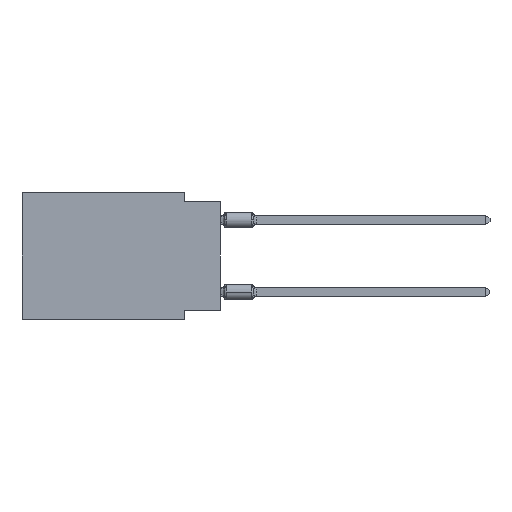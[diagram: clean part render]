
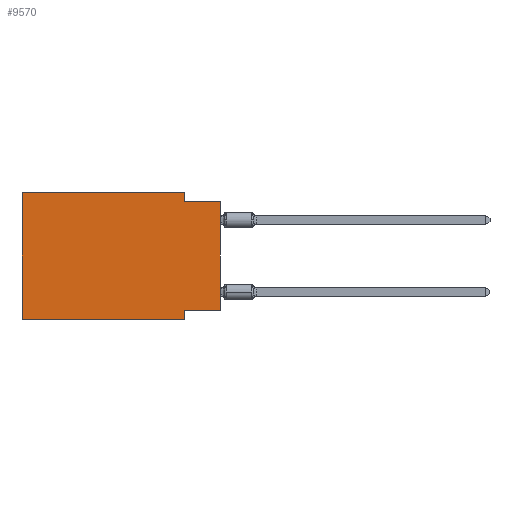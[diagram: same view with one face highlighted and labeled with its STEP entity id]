
A CAD part, left-side view. The second image highlights one B-rep face of the part: STEP entity #9570.
In plain terms, the highlighted planar face has unit normal (-1, 0, 0).
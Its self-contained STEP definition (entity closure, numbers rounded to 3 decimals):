
#768 = CARTESIAN_POINT ( 'NONE',  ( 0., 13.97, 0. ) ) ;
#900 = CARTESIAN_POINT ( 'NONE',  ( 0., 2.54, 0. ) ) ;
#932 = LINE ( 'NONE', #15008, #1315 ) ;
#1315 = VECTOR ( 'NONE', #7063, 1000. ) ;
#1549 = DIRECTION ( 'NONE',  ( 0., -1., 0. ) ) ;
#1816 = AXIS2_PLACEMENT_3D ( 'NONE', #18337, #7657, #9060 ) ;
#2041 = VERTEX_POINT ( 'NONE', #4315 ) ;
#2295 = CARTESIAN_POINT ( 'NONE',  ( 0., 2.54, -8.89 ) ) ;
#2368 = DIRECTION ( 'NONE',  ( 0., 1., 0. ) ) ;
#3233 = PLANE ( 'NONE',  #1816 ) ;
#3488 = CARTESIAN_POINT ( 'NONE',  ( 0., 13.97, 0. ) ) ;
#3851 = VECTOR ( 'NONE', #19462, 1000. ) ;
#3869 = LINE ( 'NONE', #14840, #6607 ) ;
#3931 = ORIENTED_EDGE ( 'NONE', *, *, #19091, .F. ) ;
#4048 = CARTESIAN_POINT ( 'NONE',  ( 0., 0., 0. ) ) ;
#4058 = VECTOR ( 'NONE', #15773, 1000. ) ;
#4315 = CARTESIAN_POINT ( 'NONE',  ( 0., 13.97, -8.89 ) ) ;
#4895 = CARTESIAN_POINT ( 'NONE',  ( 0., 0., -0.635 ) ) ;
#5676 = ORIENTED_EDGE ( 'NONE', *, *, #15116, .F. ) ;
#6261 = DIRECTION ( 'NONE',  ( 0., 0., 1. ) ) ;
#6607 = VECTOR ( 'NONE', #2368, 1000. ) ;
#6780 = VERTEX_POINT ( 'NONE', #18927 ) ;
#7063 = DIRECTION ( 'NONE',  ( 0., 0., -1. ) ) ;
#7137 = VERTEX_POINT ( 'NONE', #4895 ) ;
#7657 = DIRECTION ( 'NONE',  ( 1., 0., 0. ) ) ;
#7780 = EDGE_CURVE ( 'NONE', #6780, #7137, #18151, .T. ) ;
#7879 = CARTESIAN_POINT ( 'NONE',  ( 0., 13.97, -8.89 ) ) ;
#8429 = ORIENTED_EDGE ( 'NONE', *, *, #9054, .F. ) ;
#8625 = CARTESIAN_POINT ( 'NONE',  ( 0., 2.54, -0.635 ) ) ;
#9054 = EDGE_CURVE ( 'NONE', #2041, #17340, #16746, .T. ) ;
#9055 = EDGE_CURVE ( 'NONE', #15854, #7137, #12306, .T. ) ;
#9060 = DIRECTION ( 'NONE',  ( 0., 0., -1. ) ) ;
#9080 = CARTESIAN_POINT ( 'NONE',  ( 0., 0., -0.635 ) ) ;
#9570 = ADVANCED_FACE ( 'NONE', ( #10580 ), #3233, .F. ) ;
#9625 = LINE ( 'NONE', #3488, #4058 ) ;
#10580 = FACE_OUTER_BOUND ( 'NONE', #14536, .T. ) ;
#10827 = VECTOR ( 'NONE', #1549, 1000. ) ;
#10829 = ORIENTED_EDGE ( 'NONE', *, *, #13932, .F. ) ;
#10888 = VERTEX_POINT ( 'NONE', #900 ) ;
#11220 = VECTOR ( 'NONE', #19769, 1000. ) ;
#11336 = EDGE_CURVE ( 'NONE', #2041, #14540, #19764, .T. ) ;
#11811 = LINE ( 'NONE', #18161, #11220 ) ;
#12306 = LINE ( 'NONE', #9080, #10827 ) ;
#12354 = ORIENTED_EDGE ( 'NONE', *, *, #7780, .T. ) ;
#12973 = ORIENTED_EDGE ( 'NONE', *, *, #11336, .T. ) ;
#13932 = EDGE_CURVE ( 'NONE', #10888, #15854, #932, .T. ) ;
#14282 = VECTOR ( 'NONE', #16749, 1000. ) ;
#14536 = EDGE_LOOP ( 'NONE', ( #12354, #18078, #10829, #17595, #8429, #12973, #3931, #5676 ) ) ;
#14540 = VERTEX_POINT ( 'NONE', #2295 ) ;
#14840 = CARTESIAN_POINT ( 'NONE',  ( 0., 0., -8.255 ) ) ;
#15008 = CARTESIAN_POINT ( 'NONE',  ( 0., 2.54, 0. ) ) ;
#15116 = EDGE_CURVE ( 'NONE', #6780, #19460, #3869, .T. ) ;
#15225 = CARTESIAN_POINT ( 'NONE',  ( 0., 13.97, 0. ) ) ;
#15773 = DIRECTION ( 'NONE',  ( 0., -1., 0. ) ) ;
#15854 = VERTEX_POINT ( 'NONE', #8625 ) ;
#16178 = EDGE_CURVE ( 'NONE', #17340, #10888, #9625, .T. ) ;
#16221 = CARTESIAN_POINT ( 'NONE',  ( 0., 2.54, -8.255 ) ) ;
#16304 = VECTOR ( 'NONE', #6261, 1000. ) ;
#16746 = LINE ( 'NONE', #15225, #16304 ) ;
#16749 = DIRECTION ( 'NONE',  ( 0., -1., 0. ) ) ;
#17340 = VERTEX_POINT ( 'NONE', #768 ) ;
#17595 = ORIENTED_EDGE ( 'NONE', *, *, #16178, .F. ) ;
#18078 = ORIENTED_EDGE ( 'NONE', *, *, #9055, .F. ) ;
#18151 = LINE ( 'NONE', #4048, #3851 ) ;
#18161 = CARTESIAN_POINT ( 'NONE',  ( 0., 2.54, -8.89 ) ) ;
#18337 = CARTESIAN_POINT ( 'NONE',  ( 0., 13.97, 0. ) ) ;
#18927 = CARTESIAN_POINT ( 'NONE',  ( 0., 0., -8.255 ) ) ;
#19091 = EDGE_CURVE ( 'NONE', #19460, #14540, #11811, .T. ) ;
#19460 = VERTEX_POINT ( 'NONE', #16221 ) ;
#19462 = DIRECTION ( 'NONE',  ( 0., 0., 1. ) ) ;
#19764 = LINE ( 'NONE', #7879, #14282 ) ;
#19769 = DIRECTION ( 'NONE',  ( 0., 0., -1. ) ) ;
